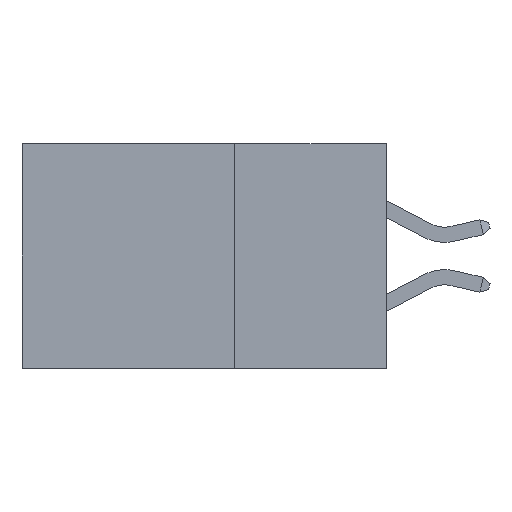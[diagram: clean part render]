
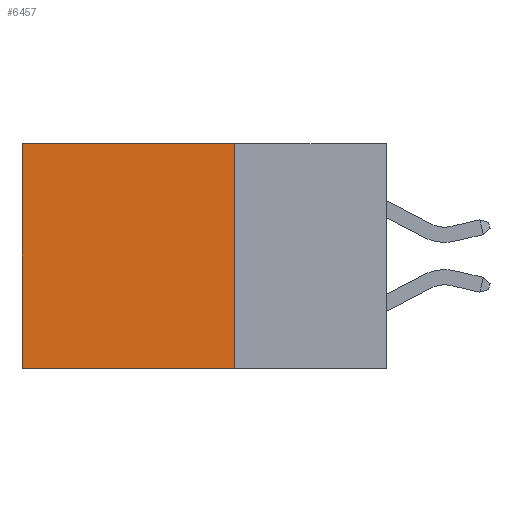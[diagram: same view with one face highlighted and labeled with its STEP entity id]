
A CAD part, left-side view. The second image highlights one B-rep face of the part: STEP entity #6457.
In plain terms, the highlighted planar face has unit normal (-1, 0, 0).
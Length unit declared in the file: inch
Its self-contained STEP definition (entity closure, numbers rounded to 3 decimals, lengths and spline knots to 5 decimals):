
#593 = DIRECTION ( 'NONE',  ( 0., 1., 0. ) ) ;
#1085 = CARTESIAN_POINT ( 'NONE',  ( 0.298, 0.6, 0. ) ) ;
#1294 = VECTOR ( 'NONE', #7666, 39.37008 ) ;
#1515 = LINE ( 'NONE', #8752, #4181 ) ;
#1603 = DIRECTION ( 'NONE',  ( 0., 0., -1. ) ) ;
#2485 = VERTEX_POINT ( 'NONE', #4448 ) ;
#2607 = DIRECTION ( 'NONE',  ( 0., 0., -1. ) ) ;
#2761 = CARTESIAN_POINT ( 'NONE',  ( 0.298, 0.25, 0. ) ) ;
#2959 = ORIENTED_EDGE ( 'NONE', *, *, #8701, .T. ) ;
#3072 = LINE ( 'NONE', #14615, #1294 ) ;
#3151 = AXIS2_PLACEMENT_3D ( 'NONE', #12913, #10628, #1603 ) ;
#3731 = EDGE_LOOP ( 'NONE', ( #2959, #11994, #9381, #12290 ) ) ;
#3861 = CARTESIAN_POINT ( 'NONE',  ( 0.298, 0.25, -0.37 ) ) ;
#4054 = VERTEX_POINT ( 'NONE', #2761 ) ;
#4181 = VECTOR ( 'NONE', #593, 39.37008 ) ;
#4448 = CARTESIAN_POINT ( 'NONE',  ( 0.298, 0.6, -0.37 ) ) ;
#5406 = DIRECTION ( 'NONE',  ( 0., 0., -1. ) ) ;
#5582 = CARTESIAN_POINT ( 'NONE',  ( 0.298, 0.6, 0. ) ) ;
#6457 = ADVANCED_FACE ( 'NONE', ( #13913 ), #13015, .F. ) ;
#6471 = CARTESIAN_POINT ( 'NONE',  ( 0.298, 0.25, 0. ) ) ;
#6532 = LINE ( 'NONE', #5582, #8144 ) ;
#7026 = VECTOR ( 'NONE', #5406, 39.37008 ) ;
#7666 = DIRECTION ( 'NONE',  ( 0., 1., 0. ) ) ;
#7949 = LINE ( 'NONE', #6471, #7026 ) ;
#8144 = VECTOR ( 'NONE', #2607, 39.37008 ) ;
#8701 = EDGE_CURVE ( 'NONE', #13404, #2485, #6532, .T. ) ;
#8752 = CARTESIAN_POINT ( 'NONE',  ( 0.298, 0.25, 0. ) ) ;
#9183 = EDGE_CURVE ( 'NONE', #4054, #11150, #7949, .T. ) ;
#9381 = ORIENTED_EDGE ( 'NONE', *, *, #9183, .F. ) ;
#10216 = EDGE_CURVE ( 'NONE', #4054, #13404, #1515, .T. ) ;
#10628 = DIRECTION ( 'NONE',  ( 1., 0., 0. ) ) ;
#11150 = VERTEX_POINT ( 'NONE', #3861 ) ;
#11791 = EDGE_CURVE ( 'NONE', #11150, #2485, #3072, .T. ) ;
#11994 = ORIENTED_EDGE ( 'NONE', *, *, #11791, .F. ) ;
#12290 = ORIENTED_EDGE ( 'NONE', *, *, #10216, .T. ) ;
#12913 = CARTESIAN_POINT ( 'NONE',  ( 0.298, 0.25, 0. ) ) ;
#13015 = PLANE ( 'NONE',  #3151 ) ;
#13404 = VERTEX_POINT ( 'NONE', #1085 ) ;
#13913 = FACE_OUTER_BOUND ( 'NONE', #3731, .T. ) ;
#14615 = CARTESIAN_POINT ( 'NONE',  ( 0.298, 0.25, -0.37 ) ) ;
